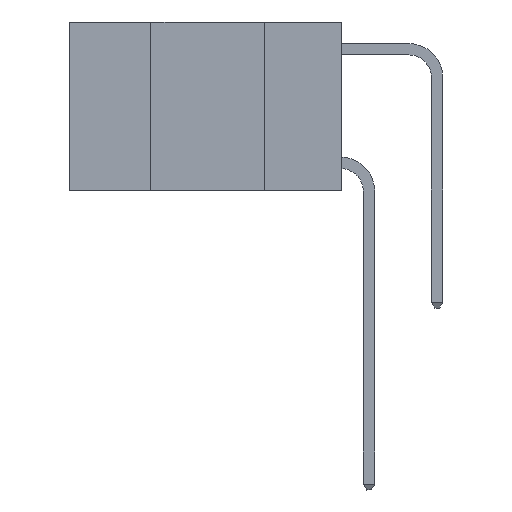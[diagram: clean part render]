
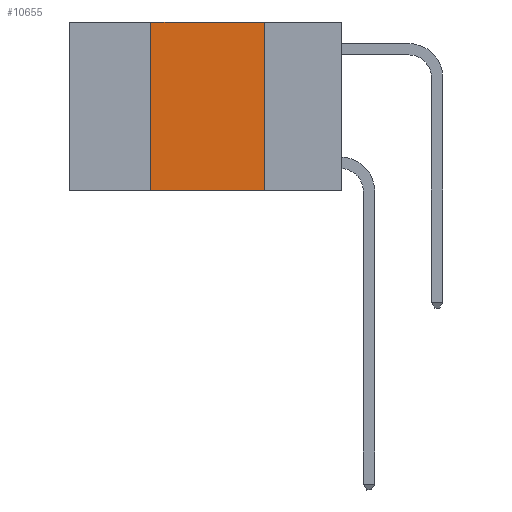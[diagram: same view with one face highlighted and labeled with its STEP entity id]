
A CAD part, left-side view. The second image highlights one B-rep face of the part: STEP entity #10655.
In plain terms, the highlighted planar face has unit normal (-1, 0, 0).
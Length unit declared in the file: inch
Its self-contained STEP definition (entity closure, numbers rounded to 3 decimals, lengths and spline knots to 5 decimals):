
#1300 = CARTESIAN_POINT ( 'NONE',  ( 0., 0.6, -0.37 ) ) ;
#1433 = VERTEX_POINT ( 'NONE', #2349 ) ;
#1439 = ORIENTED_EDGE ( 'NONE', *, *, #5844, .F. ) ;
#1468 = CARTESIAN_POINT ( 'NONE',  ( 0., 0.42, 0. ) ) ;
#1665 = ORIENTED_EDGE ( 'NONE', *, *, #1736, .F. ) ;
#1736 = EDGE_CURVE ( 'NONE', #5749, #1433, #4357, .T. ) ;
#1780 = CARTESIAN_POINT ( 'NONE',  ( 0., 0.17, 0. ) ) ;
#1788 = CARTESIAN_POINT ( 'NONE',  ( 0., 0.42, 0. ) ) ;
#1855 = LINE ( 'NONE', #1300, #6062 ) ;
#2149 = LINE ( 'NONE', #2800, #11167 ) ;
#2349 = CARTESIAN_POINT ( 'NONE',  ( 0., 0.17, -0.37 ) ) ;
#2433 = DIRECTION ( 'NONE',  ( 0., 0., 1. ) ) ;
#2800 = CARTESIAN_POINT ( 'NONE',  ( 0., 0.6, 0. ) ) ;
#3682 = VECTOR ( 'NONE', #2433, 39.37008 ) ;
#4089 = PLANE ( 'NONE',  #6548 ) ;
#4213 = VERTEX_POINT ( 'NONE', #1788 ) ;
#4357 = LINE ( 'NONE', #6085, #8993 ) ;
#4645 = DIRECTION ( 'NONE',  ( 0., -1., 0. ) ) ;
#4992 = DIRECTION ( 'NONE',  ( 0., 0., -1. ) ) ;
#5429 = EDGE_CURVE ( 'NONE', #9283, #1433, #1855, .T. ) ;
#5595 = DIRECTION ( 'NONE',  ( 0., 0., -1. ) ) ;
#5749 = VERTEX_POINT ( 'NONE', #1780 ) ;
#5844 = EDGE_CURVE ( 'NONE', #4213, #5749, #2149, .T. ) ;
#6062 = VECTOR ( 'NONE', #11032, 39.37008 ) ;
#6085 = CARTESIAN_POINT ( 'NONE',  ( 0., 0.17, 0. ) ) ;
#6548 = AXIS2_PLACEMENT_3D ( 'NONE', #7557, #10209, #4992 ) ;
#6690 = FACE_OUTER_BOUND ( 'NONE', #10453, .T. ) ;
#6967 = ORIENTED_EDGE ( 'NONE', *, *, #5429, .T. ) ;
#7557 = CARTESIAN_POINT ( 'NONE',  ( 0., 0.6, 0. ) ) ;
#8323 = LINE ( 'NONE', #1468, #3682 ) ;
#8993 = VECTOR ( 'NONE', #5595, 39.37008 ) ;
#9283 = VERTEX_POINT ( 'NONE', #11562 ) ;
#9363 = ORIENTED_EDGE ( 'NONE', *, *, #10055, .F. ) ;
#10055 = EDGE_CURVE ( 'NONE', #9283, #4213, #8323, .T. ) ;
#10209 = DIRECTION ( 'NONE',  ( 1., 0., 0. ) ) ;
#10453 = EDGE_LOOP ( 'NONE', ( #1665, #1439, #9363, #6967 ) ) ;
#10655 = ADVANCED_FACE ( 'NONE', ( #6690 ), #4089, .F. ) ;
#11032 = DIRECTION ( 'NONE',  ( 0., -1., 0. ) ) ;
#11167 = VECTOR ( 'NONE', #4645, 39.37008 ) ;
#11562 = CARTESIAN_POINT ( 'NONE',  ( 0., 0.42, -0.37 ) ) ;
